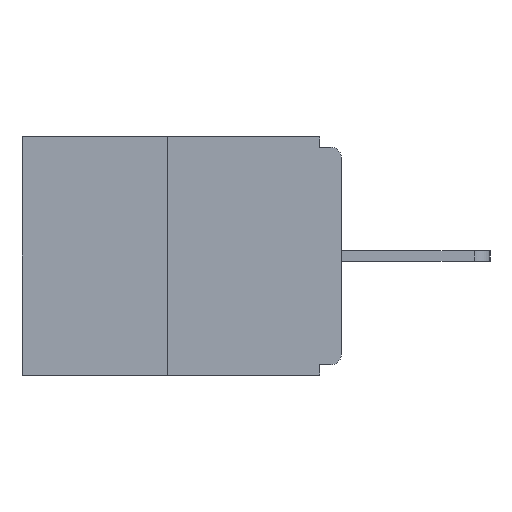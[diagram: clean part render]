
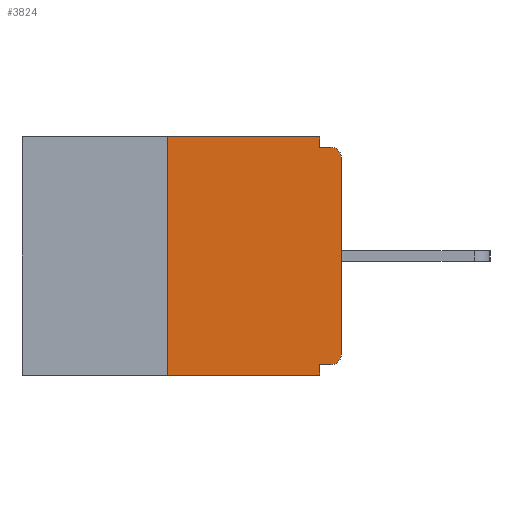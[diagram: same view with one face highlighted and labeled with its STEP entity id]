
A CAD part, left-side view. The second image highlights one B-rep face of the part: STEP entity #3824.
In plain terms, the highlighted planar face has unit normal (-1, 0, 0).
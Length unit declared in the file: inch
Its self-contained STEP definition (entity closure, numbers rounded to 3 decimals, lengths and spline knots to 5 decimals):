
#42 = CARTESIAN_POINT ( 'NONE',  ( 0., 0.015, -0.313 ) ) ;
#234 = DIRECTION ( 'NONE',  ( 0., 0., -1. ) ) ;
#239 = CIRCLE ( 'NONE', #8184, 0.015 ) ;
#277 = EDGE_CURVE ( 'NONE', #5280, #9099, #9519, .T. ) ;
#279 = CARTESIAN_POINT ( 'NONE',  ( 0., 0., -0.03 ) ) ;
#346 = VECTOR ( 'NONE', #234, 39.37008 ) ;
#366 = DIRECTION ( 'NONE',  ( 0., 0., 1. ) ) ;
#455 = ORIENTED_EDGE ( 'NONE', *, *, #277, .F. ) ;
#1109 = DIRECTION ( 'NONE',  ( 0., 0., -1. ) ) ;
#1134 = ORIENTED_EDGE ( 'NONE', *, *, #2873, .T. ) ;
#1672 = EDGE_CURVE ( 'NONE', #5939, #3474, #8355, .T. ) ;
#1793 = VERTEX_POINT ( 'NONE', #3947 ) ;
#1799 = DIRECTION ( 'NONE',  ( 0., 0., -1. ) ) ;
#1970 = VECTOR ( 'NONE', #9209, 39.37008 ) ;
#1985 = VECTOR ( 'NONE', #366, 39.37008 ) ;
#2238 = CARTESIAN_POINT ( 'NONE',  ( 0., 0.25, 0. ) ) ;
#2501 = EDGE_CURVE ( 'NONE', #8495, #5280, #7462, .T. ) ;
#2555 = CARTESIAN_POINT ( 'NONE',  ( 0., 0.25, -0.343 ) ) ;
#2715 = AXIS2_PLACEMENT_3D ( 'NONE', #9776, #10993, #9385 ) ;
#2717 = VERTEX_POINT ( 'NONE', #279 ) ;
#2815 = LINE ( 'NONE', #10326, #4606 ) ;
#2873 = EDGE_CURVE ( 'NONE', #8495, #11568, #2815, .T. ) ;
#3056 = LINE ( 'NONE', #3155, #5405 ) ;
#3155 = CARTESIAN_POINT ( 'NONE',  ( 0., 0., -0.015 ) ) ;
#3270 = LINE ( 'NONE', #10051, #346 ) ;
#3282 = LINE ( 'NONE', #11626, #5848 ) ;
#3374 = VECTOR ( 'NONE', #9707, 39.37008 ) ;
#3474 = VERTEX_POINT ( 'NONE', #12138 ) ;
#3599 = EDGE_CURVE ( 'NONE', #1793, #2717, #3282, .T. ) ;
#3824 = ADVANCED_FACE ( 'NONE', ( #9092 ), #9441, .F. ) ;
#3884 = EDGE_CURVE ( 'NONE', #9099, #8510, #3270, .T. ) ;
#3947 = CARTESIAN_POINT ( 'NONE',  ( 0., 0., -0.313 ) ) ;
#4019 = LINE ( 'NONE', #11112, #10896 ) ;
#4020 = VERTEX_POINT ( 'NONE', #8464 ) ;
#4424 = ORIENTED_EDGE ( 'NONE', *, *, #10944, .T. ) ;
#4606 = VECTOR ( 'NONE', #9001, 39.37008 ) ;
#4854 = ORIENTED_EDGE ( 'NONE', *, *, #7215, .F. ) ;
#5280 = VERTEX_POINT ( 'NONE', #5657 ) ;
#5405 = VECTOR ( 'NONE', #6047, 39.37008 ) ;
#5657 = CARTESIAN_POINT ( 'NONE',  ( 0., 0.25, 0. ) ) ;
#5848 = VECTOR ( 'NONE', #11648, 39.37008 ) ;
#5904 = DIRECTION ( 'NONE',  ( -1., 0., 0. ) ) ;
#5939 = VERTEX_POINT ( 'NONE', #8979 ) ;
#6021 = CARTESIAN_POINT ( 'NONE',  ( 0., 0., -0.328 ) ) ;
#6047 = DIRECTION ( 'NONE',  ( 0., -1., 0. ) ) ;
#6204 = ORIENTED_EDGE ( 'NONE', *, *, #2501, .F. ) ;
#6291 = CARTESIAN_POINT ( 'NONE',  ( 0., 0.46, 0. ) ) ;
#6668 = ORIENTED_EDGE ( 'NONE', *, *, #8654, .F. ) ;
#7101 = DIRECTION ( 'NONE',  ( -1., 0., 0. ) ) ;
#7215 = EDGE_CURVE ( 'NONE', #8510, #4020, #3056, .T. ) ;
#7462 = LINE ( 'NONE', #2238, #1985 ) ;
#7869 = CARTESIAN_POINT ( 'NONE',  ( 0., 0.031, -0.343 ) ) ;
#8001 = ORIENTED_EDGE ( 'NONE', *, *, #3599, .T. ) ;
#8082 = ORIENTED_EDGE ( 'NONE', *, *, #3884, .F. ) ;
#8184 = AXIS2_PLACEMENT_3D ( 'NONE', #11207, #5904, #12046 ) ;
#8294 = ORIENTED_EDGE ( 'NONE', *, *, #10581, .T. ) ;
#8305 = CIRCLE ( 'NONE', #11077, 0.015 ) ;
#8355 = LINE ( 'NONE', #6021, #3374 ) ;
#8464 = CARTESIAN_POINT ( 'NONE',  ( 0., 0.015, -0.015 ) ) ;
#8495 = VERTEX_POINT ( 'NONE', #2555 ) ;
#8510 = VERTEX_POINT ( 'NONE', #9204 ) ;
#8654 = EDGE_CURVE ( 'NONE', #3474, #11568, #4019, .T. ) ;
#8979 = CARTESIAN_POINT ( 'NONE',  ( 0., 0.015, -0.328 ) ) ;
#9001 = DIRECTION ( 'NONE',  ( 0., -1., 0. ) ) ;
#9092 = FACE_OUTER_BOUND ( 'NONE', #10735, .T. ) ;
#9099 = VERTEX_POINT ( 'NONE', #11595 ) ;
#9204 = CARTESIAN_POINT ( 'NONE',  ( 0., 0.031, -0.015 ) ) ;
#9209 = DIRECTION ( 'NONE',  ( 0., -1., 0. ) ) ;
#9385 = DIRECTION ( 'NONE',  ( 0., 0., -1. ) ) ;
#9441 = PLANE ( 'NONE',  #2715 ) ;
#9519 = LINE ( 'NONE', #6291, #1970 ) ;
#9707 = DIRECTION ( 'NONE',  ( 0., 1., 0. ) ) ;
#9776 = CARTESIAN_POINT ( 'NONE',  ( 0., 0.46, 0. ) ) ;
#10017 = ORIENTED_EDGE ( 'NONE', *, *, #1672, .F. ) ;
#10051 = CARTESIAN_POINT ( 'NONE',  ( 0., 0.031, 0. ) ) ;
#10326 = CARTESIAN_POINT ( 'NONE',  ( 0., 0.46, -0.343 ) ) ;
#10581 = EDGE_CURVE ( 'NONE', #2717, #4020, #239, .T. ) ;
#10735 = EDGE_LOOP ( 'NONE', ( #455, #6204, #1134, #6668, #10017, #4424, #8001, #8294, #4854, #8082 ) ) ;
#10896 = VECTOR ( 'NONE', #1799, 39.37008 ) ;
#10944 = EDGE_CURVE ( 'NONE', #5939, #1793, #8305, .T. ) ;
#10993 = DIRECTION ( 'NONE',  ( 1., 0., 0. ) ) ;
#11077 = AXIS2_PLACEMENT_3D ( 'NONE', #42, #7101, #1109 ) ;
#11112 = CARTESIAN_POINT ( 'NONE',  ( 0., 0.031, -0.343 ) ) ;
#11207 = CARTESIAN_POINT ( 'NONE',  ( 0., 0.015, -0.03 ) ) ;
#11568 = VERTEX_POINT ( 'NONE', #7869 ) ;
#11595 = CARTESIAN_POINT ( 'NONE',  ( 0., 0.031, 0. ) ) ;
#11626 = CARTESIAN_POINT ( 'NONE',  ( 0., 0., 0. ) ) ;
#11648 = DIRECTION ( 'NONE',  ( 0., 0., 1. ) ) ;
#12046 = DIRECTION ( 'NONE',  ( 0., 0., -1. ) ) ;
#12138 = CARTESIAN_POINT ( 'NONE',  ( 0., 0.031, -0.328 ) ) ;
